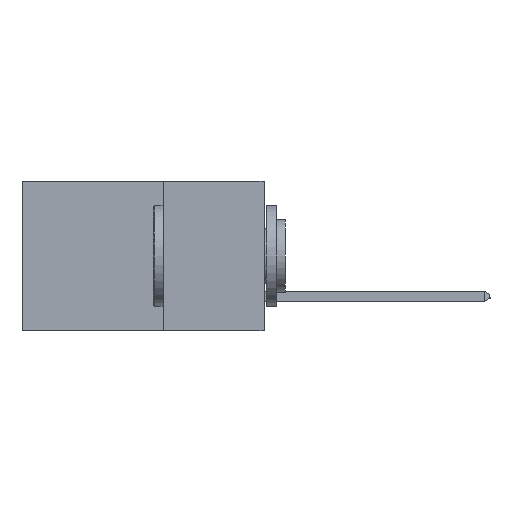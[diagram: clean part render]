
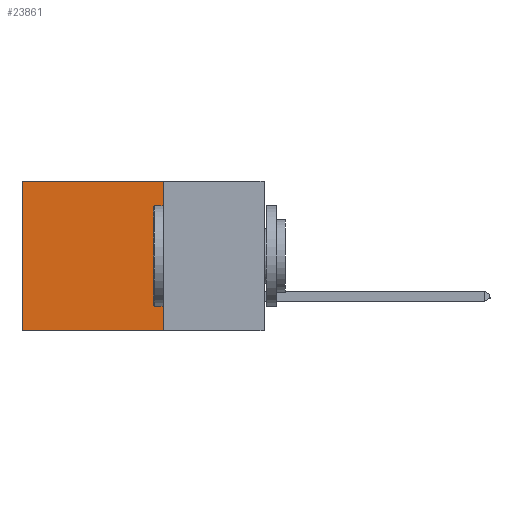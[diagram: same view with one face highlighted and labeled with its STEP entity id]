
A CAD part, left-side view. The second image highlights one B-rep face of the part: STEP entity #23861.
In plain terms, the highlighted planar face has unit normal (-1, 0, 0).
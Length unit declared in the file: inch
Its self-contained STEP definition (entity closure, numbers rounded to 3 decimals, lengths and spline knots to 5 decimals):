
#62 = VERTEX_POINT ( 'NONE', #7868 ) ;
#1287 = CARTESIAN_POINT ( 'NONE',  ( 0.298, 0.25, 0. ) ) ;
#1892 = CARTESIAN_POINT ( 'NONE',  ( 0.298, 0.6, 0. ) ) ;
#2464 = VECTOR ( 'NONE', #27276, 39.37008 ) ;
#3579 = DIRECTION ( 'NONE',  ( 0., 0., -1. ) ) ;
#3628 = AXIS2_PLACEMENT_3D ( 'NONE', #1287, #17008, #3579 ) ;
#4653 = VECTOR ( 'NONE', #16939, 39.37008 ) ;
#5841 = VERTEX_POINT ( 'NONE', #20908 ) ;
#7281 = VECTOR ( 'NONE', #21092, 39.37008 ) ;
#7868 = CARTESIAN_POINT ( 'NONE',  ( 0.298, 0.25, -0.37 ) ) ;
#8537 = LINE ( 'NONE', #22869, #2464 ) ;
#8807 = VERTEX_POINT ( 'NONE', #26262 ) ;
#9474 = VERTEX_POINT ( 'NONE', #1892 ) ;
#9929 = VECTOR ( 'NONE', #19679, 39.37008 ) ;
#9964 = ORIENTED_EDGE ( 'NONE', *, *, #20353, .F. ) ;
#14778 = CARTESIAN_POINT ( 'NONE',  ( 0.298, 0.6, 0. ) ) ;
#15065 = EDGE_CURVE ( 'NONE', #5841, #62, #20486, .T. ) ;
#15094 = ORIENTED_EDGE ( 'NONE', *, *, #20017, .T. ) ;
#16580 = LINE ( 'NONE', #14778, #4653 ) ;
#16939 = DIRECTION ( 'NONE',  ( 0., 0., -1. ) ) ;
#17008 = DIRECTION ( 'NONE',  ( 1., 0., 0. ) ) ;
#17345 = FACE_OUTER_BOUND ( 'NONE', #22734, .T. ) ;
#17487 = CARTESIAN_POINT ( 'NONE',  ( 0.298, 0.25, -0.37 ) ) ;
#19679 = DIRECTION ( 'NONE',  ( 0., 1., 0. ) ) ;
#20017 = EDGE_CURVE ( 'NONE', #5841, #9474, #8537, .T. ) ;
#20353 = EDGE_CURVE ( 'NONE', #62, #8807, #21637, .T. ) ;
#20486 = LINE ( 'NONE', #23314, #7281 ) ;
#20908 = CARTESIAN_POINT ( 'NONE',  ( 0.298, 0.25, 0. ) ) ;
#21092 = DIRECTION ( 'NONE',  ( 0., 0., -1. ) ) ;
#21594 = ORIENTED_EDGE ( 'NONE', *, *, #15065, .F. ) ;
#21637 = LINE ( 'NONE', #17487, #9929 ) ;
#22454 = ORIENTED_EDGE ( 'NONE', *, *, #25166, .T. ) ;
#22734 = EDGE_LOOP ( 'NONE', ( #22454, #9964, #21594, #15094 ) ) ;
#22869 = CARTESIAN_POINT ( 'NONE',  ( 0.298, 0.25, 0. ) ) ;
#23314 = CARTESIAN_POINT ( 'NONE',  ( 0.298, 0.25, 0. ) ) ;
#23861 = ADVANCED_FACE ( 'NONE', ( #17345 ), #25757, .F. ) ;
#25166 = EDGE_CURVE ( 'NONE', #9474, #8807, #16580, .T. ) ;
#25757 = PLANE ( 'NONE',  #3628 ) ;
#26262 = CARTESIAN_POINT ( 'NONE',  ( 0.298, 0.6, -0.37 ) ) ;
#27276 = DIRECTION ( 'NONE',  ( 0., 1., 0. ) ) ;
